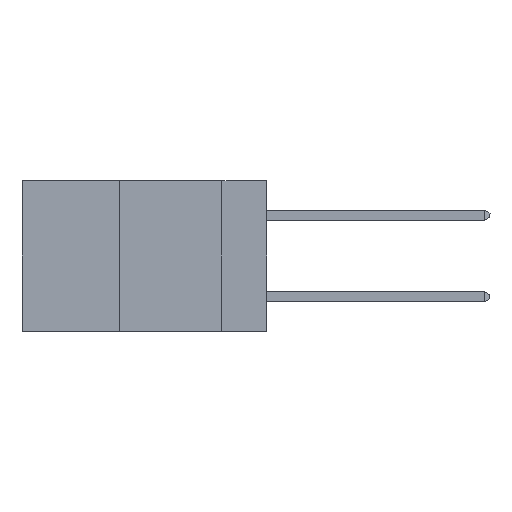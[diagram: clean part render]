
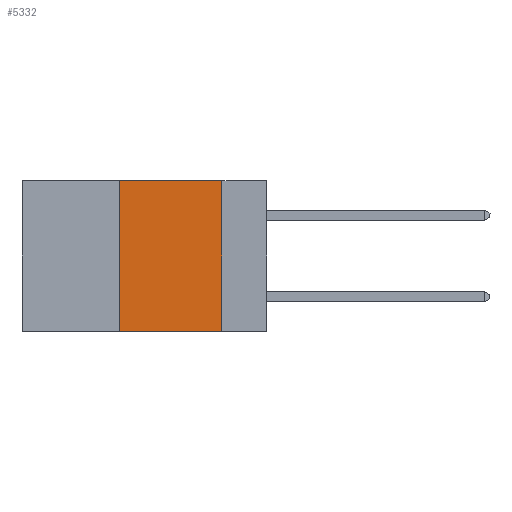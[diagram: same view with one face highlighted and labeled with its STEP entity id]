
A CAD part, left-side view. The second image highlights one B-rep face of the part: STEP entity #5332.
In plain terms, the highlighted planar face has unit normal (-1, 0, 0).
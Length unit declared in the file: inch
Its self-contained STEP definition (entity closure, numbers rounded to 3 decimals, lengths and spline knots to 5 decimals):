
#96 = ORIENTED_EDGE ( 'NONE', *, *, #13788, .F. ) ;
#232 = DIRECTION ( 'NONE',  ( 0., -1., 0. ) ) ;
#249 = CARTESIAN_POINT ( 'NONE',  ( 0., 0.11, 0. ) ) ;
#361 = CARTESIAN_POINT ( 'NONE',  ( 0., 0.36, 0. ) ) ;
#828 = LINE ( 'NONE', #2116, #7369 ) ;
#1567 = AXIS2_PLACEMENT_3D ( 'NONE', #9303, #1964, #10453 ) ;
#1964 = DIRECTION ( 'NONE',  ( 1., 0., 0. ) ) ;
#2116 = CARTESIAN_POINT ( 'NONE',  ( 0., 0.11, 0. ) ) ;
#2462 = LINE ( 'NONE', #13826, #12018 ) ;
#2829 = LINE ( 'NONE', #7028, #5746 ) ;
#3342 = DIRECTION ( 'NONE',  ( 0., 0., -1. ) ) ;
#3581 = FACE_OUTER_BOUND ( 'NONE', #13920, .T. ) ;
#3666 = VERTEX_POINT ( 'NONE', #3817 ) ;
#3765 = VERTEX_POINT ( 'NONE', #361 ) ;
#3817 = CARTESIAN_POINT ( 'NONE',  ( 0., 0.36, -0.37 ) ) ;
#4765 = LINE ( 'NONE', #8803, #13794 ) ;
#5297 = VERTEX_POINT ( 'NONE', #12571 ) ;
#5332 = ADVANCED_FACE ( 'NONE', ( #3581 ), #15044, .F. ) ;
#5412 = EDGE_CURVE ( 'NONE', #3666, #3765, #2829, .T. ) ;
#5746 = VECTOR ( 'NONE', #5824, 39.37008 ) ;
#5824 = DIRECTION ( 'NONE',  ( 0., 0., 1. ) ) ;
#6271 = ORIENTED_EDGE ( 'NONE', *, *, #10975, .F. ) ;
#7028 = CARTESIAN_POINT ( 'NONE',  ( 0., 0.36, 0. ) ) ;
#7369 = VECTOR ( 'NONE', #3342, 39.37008 ) ;
#8041 = DIRECTION ( 'NONE',  ( 0., -1., 0. ) ) ;
#8619 = EDGE_CURVE ( 'NONE', #3666, #5297, #4765, .T. ) ;
#8803 = CARTESIAN_POINT ( 'NONE',  ( 0., 0.6, -0.37 ) ) ;
#9303 = CARTESIAN_POINT ( 'NONE',  ( 0., 0.6, 0. ) ) ;
#10453 = DIRECTION ( 'NONE',  ( 0., 0., -1. ) ) ;
#10975 = EDGE_CURVE ( 'NONE', #13575, #5297, #828, .T. ) ;
#12018 = VECTOR ( 'NONE', #8041, 39.37008 ) ;
#12571 = CARTESIAN_POINT ( 'NONE',  ( 0., 0.11, -0.37 ) ) ;
#12843 = ORIENTED_EDGE ( 'NONE', *, *, #5412, .F. ) ;
#13575 = VERTEX_POINT ( 'NONE', #249 ) ;
#13788 = EDGE_CURVE ( 'NONE', #3765, #13575, #2462, .T. ) ;
#13794 = VECTOR ( 'NONE', #232, 39.37008 ) ;
#13826 = CARTESIAN_POINT ( 'NONE',  ( 0., 0.6, 0. ) ) ;
#13920 = EDGE_LOOP ( 'NONE', ( #6271, #96, #12843, #13950 ) ) ;
#13950 = ORIENTED_EDGE ( 'NONE', *, *, #8619, .T. ) ;
#15044 = PLANE ( 'NONE',  #1567 ) ;
